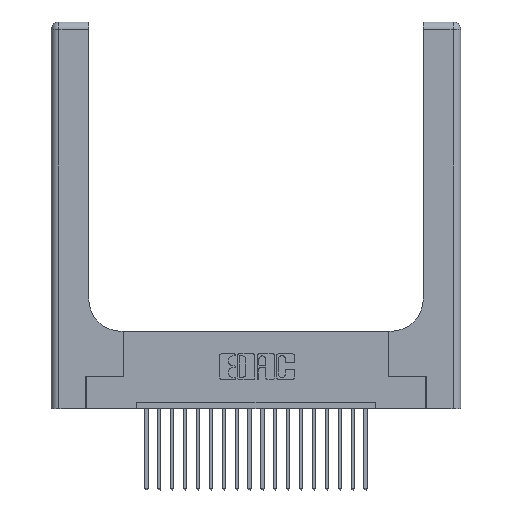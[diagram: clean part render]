
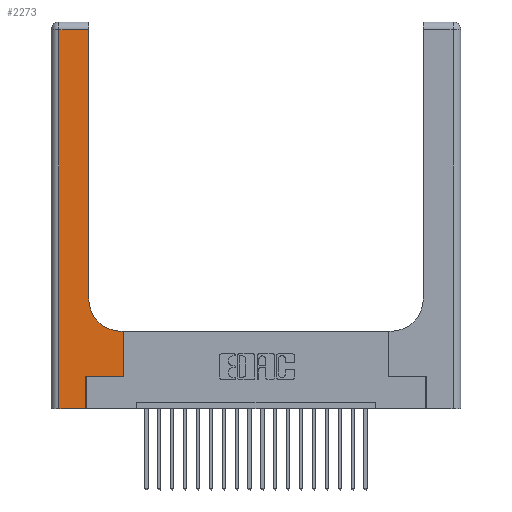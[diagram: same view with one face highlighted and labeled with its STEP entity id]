
A CAD part, top view. The second image highlights one B-rep face of the part: STEP entity #2273.
In plain terms, the highlighted planar face has unit normal (0, 0, 1).
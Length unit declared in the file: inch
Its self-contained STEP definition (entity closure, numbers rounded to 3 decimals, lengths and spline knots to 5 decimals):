
#45 = DIRECTION ( 'NONE',  ( -1., 0., 0. ) ) ;
#366 = EDGE_CURVE ( 'NONE', #10480, #13833, #20737, .T. ) ;
#687 = CARTESIAN_POINT ( 'NONE',  ( 0.5415, 0.6, 0.37 ) ) ;
#1191 = CARTESIAN_POINT ( 'NONE',  ( 0.2915, 2.94, 0.37 ) ) ;
#1280 = FACE_OUTER_BOUND ( 'NONE', #4448, .T. ) ;
#1488 = DIRECTION ( 'NONE',  ( -1., 0., 0. ) ) ;
#1874 = CARTESIAN_POINT ( 'NONE',  ( 0.269, 0., 0.37 ) ) ;
#1876 = VECTOR ( 'NONE', #10787, 39.37008 ) ;
#2059 = VERTEX_POINT ( 'NONE', #17287 ) ;
#2273 = ADVANCED_FACE ( 'NONE', ( #1280 ), #19281, .F. ) ;
#2599 = DIRECTION ( 'NONE',  ( -1., 0., 0. ) ) ;
#2888 = VECTOR ( 'NONE', #3598, 39.37008 ) ;
#2996 = EDGE_CURVE ( 'NONE', #6248, #11230, #8898, .T. ) ;
#3156 = CARTESIAN_POINT ( 'NONE',  ( 0.269, 0.25, 0.37 ) ) ;
#3196 = CARTESIAN_POINT ( 'NONE',  ( 0.5415, 0.85, 0.37 ) ) ;
#3345 = LINE ( 'NONE', #13273, #4386 ) ;
#3598 = DIRECTION ( 'NONE',  ( 1., 0., 0. ) ) ;
#3831 = AXIS2_PLACEMENT_3D ( 'NONE', #19428, #12761, #2599 ) ;
#4037 = ORIENTED_EDGE ( 'NONE', *, *, #14714, .T. ) ;
#4386 = VECTOR ( 'NONE', #6494, 39.37008 ) ;
#4448 = EDGE_LOOP ( 'NONE', ( #8526, #6488, #18458, #4037, #18833, #4692, #19455, #13140, #20935 ) ) ;
#4692 = ORIENTED_EDGE ( 'NONE', *, *, #10408, .T. ) ;
#4864 = DIRECTION ( 'NONE',  ( 0., 0., -1. ) ) ;
#5228 = LINE ( 'NONE', #3156, #2888 ) ;
#5288 = EDGE_CURVE ( 'NONE', #2059, #6248, #3345, .T. ) ;
#5776 = DIRECTION ( 'NONE',  ( 0., 1., 0. ) ) ;
#6084 = DIRECTION ( 'NONE',  ( 1., 0., 0. ) ) ;
#6198 = LINE ( 'NONE', #1874, #19787 ) ;
#6248 = VERTEX_POINT ( 'NONE', #1191 ) ;
#6488 = ORIENTED_EDGE ( 'NONE', *, *, #2996, .T. ) ;
#6494 = DIRECTION ( 'NONE',  ( 0., 1., 0. ) ) ;
#6915 = VERTEX_POINT ( 'NONE', #14744 ) ;
#7641 = CARTESIAN_POINT ( 'NONE',  ( 0., 0., 0.37 ) ) ;
#7673 = DIRECTION ( 'NONE',  ( 0., 1., 0. ) ) ;
#8121 = VERTEX_POINT ( 'NONE', #8826 ) ;
#8163 = EDGE_CURVE ( 'NONE', #11230, #8121, #18854, .T. ) ;
#8526 = ORIENTED_EDGE ( 'NONE', *, *, #5288, .T. ) ;
#8765 = CARTESIAN_POINT ( 'NONE',  ( 0.06, 2.94, 0.37 ) ) ;
#8826 = CARTESIAN_POINT ( 'NONE',  ( 0.06, 0., 0.37 ) ) ;
#8876 = LINE ( 'NONE', #21805, #17109 ) ;
#8898 = LINE ( 'NONE', #17220, #10531 ) ;
#9318 = VECTOR ( 'NONE', #6084, 39.37008 ) ;
#9772 = CARTESIAN_POINT ( 'NONE',  ( 0.5585, 0.25, 0.37 ) ) ;
#10051 = AXIS2_PLACEMENT_3D ( 'NONE', #3196, #4864, #11741 ) ;
#10408 = EDGE_CURVE ( 'NONE', #12429, #10480, #5228, .T. ) ;
#10480 = VERTEX_POINT ( 'NONE', #9772 ) ;
#10531 = VECTOR ( 'NONE', #45, 39.37008 ) ;
#10713 = CARTESIAN_POINT ( 'NONE',  ( 0.06, 3., 0.37 ) ) ;
#10787 = DIRECTION ( 'NONE',  ( 0., -1., 0. ) ) ;
#11230 = VERTEX_POINT ( 'NONE', #8765 ) ;
#11445 = VERTEX_POINT ( 'NONE', #687 ) ;
#11741 = DIRECTION ( 'NONE',  ( 1., 0., 0. ) ) ;
#11863 = EDGE_CURVE ( 'NONE', #11445, #2059, #13682, .T. ) ;
#12429 = VERTEX_POINT ( 'NONE', #18209 ) ;
#12671 = EDGE_CURVE ( 'NONE', #6915, #12429, #6198, .T. ) ;
#12761 = DIRECTION ( 'NONE',  ( 0., 0., -1. ) ) ;
#13051 = LINE ( 'NONE', #7641, #9318 ) ;
#13140 = ORIENTED_EDGE ( 'NONE', *, *, #20735, .T. ) ;
#13273 = CARTESIAN_POINT ( 'NONE',  ( 0.2915, 3., 0.37 ) ) ;
#13682 = CIRCLE ( 'NONE', #10051, 0.25 ) ;
#13833 = VERTEX_POINT ( 'NONE', #16953 ) ;
#14621 = VECTOR ( 'NONE', #7673, 39.37008 ) ;
#14714 = EDGE_CURVE ( 'NONE', #8121, #6915, #13051, .T. ) ;
#14744 = CARTESIAN_POINT ( 'NONE',  ( 0.269, 0., 0.37 ) ) ;
#16953 = CARTESIAN_POINT ( 'NONE',  ( 0.5585, 0.6, 0.37 ) ) ;
#17109 = VECTOR ( 'NONE', #1488, 39.37008 ) ;
#17220 = CARTESIAN_POINT ( 'NONE',  ( 0., 2.94, 0.37 ) ) ;
#17287 = CARTESIAN_POINT ( 'NONE',  ( 0.2915, 0.85, 0.37 ) ) ;
#17873 = CARTESIAN_POINT ( 'NONE',  ( 0.5585, 0.25, 0.37 ) ) ;
#18209 = CARTESIAN_POINT ( 'NONE',  ( 0.269, 0.25, 0.37 ) ) ;
#18458 = ORIENTED_EDGE ( 'NONE', *, *, #8163, .T. ) ;
#18833 = ORIENTED_EDGE ( 'NONE', *, *, #12671, .T. ) ;
#18854 = LINE ( 'NONE', #10713, #1876 ) ;
#19281 = PLANE ( 'NONE',  #3831 ) ;
#19428 = CARTESIAN_POINT ( 'NONE',  ( 0., 3., 0.37 ) ) ;
#19455 = ORIENTED_EDGE ( 'NONE', *, *, #366, .T. ) ;
#19787 = VECTOR ( 'NONE', #5776, 39.37008 ) ;
#20735 = EDGE_CURVE ( 'NONE', #13833, #11445, #8876, .T. ) ;
#20737 = LINE ( 'NONE', #17873, #14621 ) ;
#20935 = ORIENTED_EDGE ( 'NONE', *, *, #11863, .T. ) ;
#21805 = CARTESIAN_POINT ( 'NONE',  ( 0.2915, 0.6, 0.37 ) ) ;
